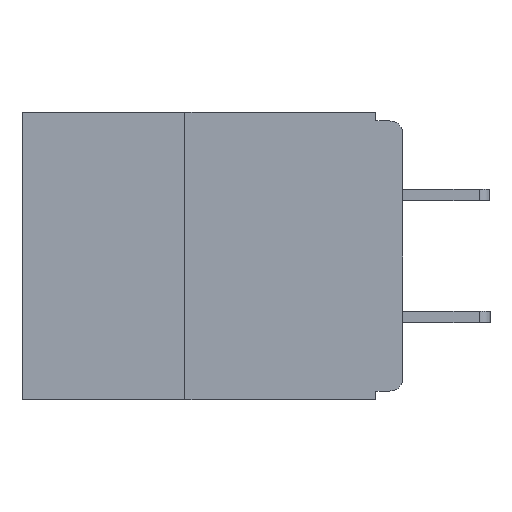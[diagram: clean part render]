
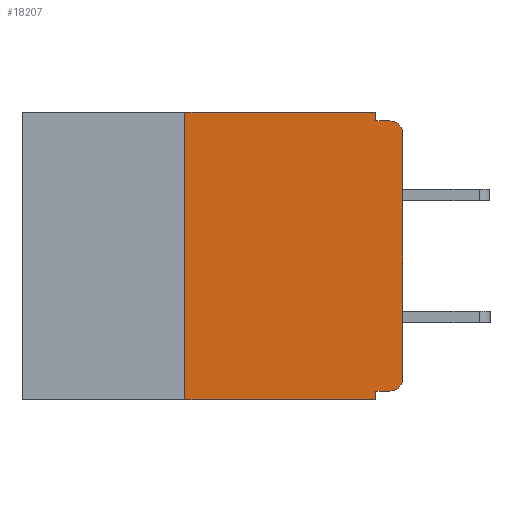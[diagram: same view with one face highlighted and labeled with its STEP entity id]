
A CAD part, left-side view. The second image highlights one B-rep face of the part: STEP entity #18207.
In plain terms, the highlighted planar face has unit normal (-1, 0, 0).
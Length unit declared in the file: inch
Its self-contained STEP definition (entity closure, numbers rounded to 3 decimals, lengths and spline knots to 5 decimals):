
#3 = VECTOR ( 'NONE', #7813, 39.37008 ) ;
#144 = EDGE_CURVE ( 'NONE', #2529, #11966, #22328, .T. ) ;
#291 = CIRCLE ( 'NONE', #22810, 0.015 ) ;
#679 = LINE ( 'NONE', #9348, #3 ) ;
#1463 = DIRECTION ( 'NONE',  ( 0., 0., -1. ) ) ;
#2529 = VERTEX_POINT ( 'NONE', #10943 ) ;
#3318 = VERTEX_POINT ( 'NONE', #25193 ) ;
#3394 = VERTEX_POINT ( 'NONE', #22913 ) ;
#3469 = EDGE_CURVE ( 'NONE', #5312, #24483, #15599, .T. ) ;
#3575 = CARTESIAN_POINT ( 'NONE',  ( 0., 0.437, 0. ) ) ;
#4626 = CARTESIAN_POINT ( 'NONE',  ( 0., 0., -0.305 ) ) ;
#4814 = CARTESIAN_POINT ( 'NONE',  ( 0., 0., -0.32 ) ) ;
#5201 = ORIENTED_EDGE ( 'NONE', *, *, #23504, .T. ) ;
#5312 = VERTEX_POINT ( 'NONE', #10881 ) ;
#5868 = DIRECTION ( 'NONE',  ( 0., 0., -1. ) ) ;
#6501 = EDGE_CURVE ( 'NONE', #11966, #3318, #679, .T. ) ;
#6586 = CARTESIAN_POINT ( 'NONE',  ( 0., 0.031, -0.33 ) ) ;
#6825 = ORIENTED_EDGE ( 'NONE', *, *, #144, .F. ) ;
#7360 = DIRECTION ( 'NONE',  ( -1., 0., 0. ) ) ;
#7752 = PLANE ( 'NONE',  #12730 ) ;
#7783 = ORIENTED_EDGE ( 'NONE', *, *, #12775, .T. ) ;
#7813 = DIRECTION ( 'NONE',  ( 0., -1., 0. ) ) ;
#8038 = CARTESIAN_POINT ( 'NONE',  ( 0., 0.437, 0. ) ) ;
#8680 = DIRECTION ( 'NONE',  ( 0., 0., -1. ) ) ;
#8682 = EDGE_CURVE ( 'NONE', #9891, #23603, #14093, .T. ) ;
#9156 = VECTOR ( 'NONE', #24941, 39.37008 ) ;
#9329 = LINE ( 'NONE', #20462, #24653 ) ;
#9348 = CARTESIAN_POINT ( 'NONE',  ( 0., 0., -0.01 ) ) ;
#9743 = VECTOR ( 'NONE', #8680, 39.37008 ) ;
#9891 = VERTEX_POINT ( 'NONE', #17487 ) ;
#10035 = ORIENTED_EDGE ( 'NONE', *, *, #21156, .T. ) ;
#10881 = CARTESIAN_POINT ( 'NONE',  ( 0., 0.25, -0.33 ) ) ;
#10943 = CARTESIAN_POINT ( 'NONE',  ( 0., 0.031, 0. ) ) ;
#11338 = ORIENTED_EDGE ( 'NONE', *, *, #17894, .F. ) ;
#11491 = VECTOR ( 'NONE', #20400, 39.37008 ) ;
#11692 = EDGE_CURVE ( 'NONE', #24483, #2529, #22694, .T. ) ;
#11879 = DIRECTION ( 'NONE',  ( 0., 0., -1. ) ) ;
#11966 = VERTEX_POINT ( 'NONE', #22985 ) ;
#12730 = AXIS2_PLACEMENT_3D ( 'NONE', #3575, #23811, #11879 ) ;
#12775 = EDGE_CURVE ( 'NONE', #15865, #3318, #291, .T. ) ;
#12942 = FACE_OUTER_BOUND ( 'NONE', #19380, .T. ) ;
#13115 = DIRECTION ( 'NONE',  ( 0., 1., 0. ) ) ;
#13261 = ORIENTED_EDGE ( 'NONE', *, *, #6501, .F. ) ;
#13281 = ORIENTED_EDGE ( 'NONE', *, *, #26127, .F. ) ;
#13806 = DIRECTION ( 'NONE',  ( -1., 0., 0. ) ) ;
#14093 = CIRCLE ( 'NONE', #17277, 0.015 ) ;
#14564 = ORIENTED_EDGE ( 'NONE', *, *, #8682, .T. ) ;
#15093 = CARTESIAN_POINT ( 'NONE',  ( 0., 0.031, 0. ) ) ;
#15599 = LINE ( 'NONE', #20314, #11491 ) ;
#15865 = VERTEX_POINT ( 'NONE', #22546 ) ;
#17028 = VECTOR ( 'NONE', #5868, 39.37008 ) ;
#17277 = AXIS2_PLACEMENT_3D ( 'NONE', #25613, #13806, #1463 ) ;
#17283 = VECTOR ( 'NONE', #13115, 39.37008 ) ;
#17487 = CARTESIAN_POINT ( 'NONE',  ( 0., 0.015, -0.32 ) ) ;
#17894 = EDGE_CURVE ( 'NONE', #22358, #3394, #25620, .T. ) ;
#18207 = ADVANCED_FACE ( 'NONE', ( #12942 ), #7752, .F. ) ;
#18218 = DIRECTION ( 'NONE',  ( 0., -1., 0. ) ) ;
#18533 = DIRECTION ( 'NONE',  ( 0., -1., 0. ) ) ;
#19028 = CARTESIAN_POINT ( 'NONE',  ( 0., 0., 0. ) ) ;
#19267 = LINE ( 'NONE', #19028, #9156 ) ;
#19380 = EDGE_LOOP ( 'NONE', ( #10035, #7783, #13261, #6825, #23513, #19520, #5201, #11338, #13281, #14564 ) ) ;
#19490 = CARTESIAN_POINT ( 'NONE',  ( 0., 0.015, -0.025 ) ) ;
#19520 = ORIENTED_EDGE ( 'NONE', *, *, #3469, .F. ) ;
#20314 = CARTESIAN_POINT ( 'NONE',  ( 0., 0.25, -0.33 ) ) ;
#20400 = DIRECTION ( 'NONE',  ( 0., 0., 1. ) ) ;
#20462 = CARTESIAN_POINT ( 'NONE',  ( 0., 0.437, -0.33 ) ) ;
#21156 = EDGE_CURVE ( 'NONE', #23603, #15865, #19267, .T. ) ;
#21484 = DIRECTION ( 'NONE',  ( 0., 0., -1. ) ) ;
#21697 = CARTESIAN_POINT ( 'NONE',  ( 0., 0.25, 0. ) ) ;
#22073 = VECTOR ( 'NONE', #18218, 39.37008 ) ;
#22328 = LINE ( 'NONE', #15093, #17028 ) ;
#22358 = VERTEX_POINT ( 'NONE', #23035 ) ;
#22546 = CARTESIAN_POINT ( 'NONE',  ( 0., 0., -0.025 ) ) ;
#22593 = LINE ( 'NONE', #4814, #17283 ) ;
#22694 = LINE ( 'NONE', #8038, #22073 ) ;
#22810 = AXIS2_PLACEMENT_3D ( 'NONE', #19490, #7360, #21484 ) ;
#22913 = CARTESIAN_POINT ( 'NONE',  ( 0., 0.031, -0.33 ) ) ;
#22985 = CARTESIAN_POINT ( 'NONE',  ( 0., 0.031, -0.01 ) ) ;
#23035 = CARTESIAN_POINT ( 'NONE',  ( 0., 0.031, -0.32 ) ) ;
#23504 = EDGE_CURVE ( 'NONE', #5312, #3394, #9329, .T. ) ;
#23513 = ORIENTED_EDGE ( 'NONE', *, *, #11692, .F. ) ;
#23603 = VERTEX_POINT ( 'NONE', #4626 ) ;
#23811 = DIRECTION ( 'NONE',  ( 1., 0., 0. ) ) ;
#24483 = VERTEX_POINT ( 'NONE', #21697 ) ;
#24653 = VECTOR ( 'NONE', #18533, 39.37008 ) ;
#24941 = DIRECTION ( 'NONE',  ( 0., 0., 1. ) ) ;
#25193 = CARTESIAN_POINT ( 'NONE',  ( 0., 0.015, -0.01 ) ) ;
#25613 = CARTESIAN_POINT ( 'NONE',  ( 0., 0.015, -0.305 ) ) ;
#25620 = LINE ( 'NONE', #6586, #9743 ) ;
#26127 = EDGE_CURVE ( 'NONE', #9891, #22358, #22593, .T. ) ;
